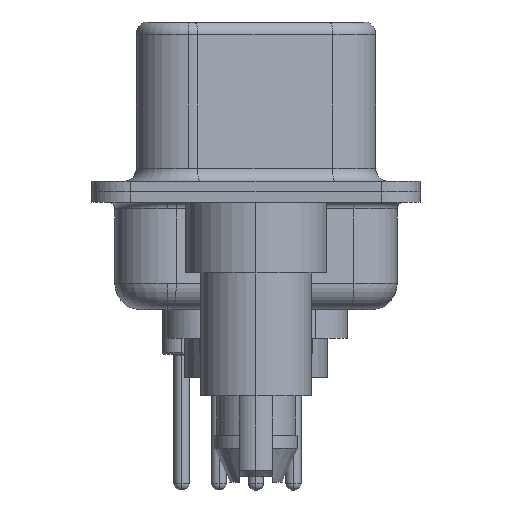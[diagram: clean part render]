
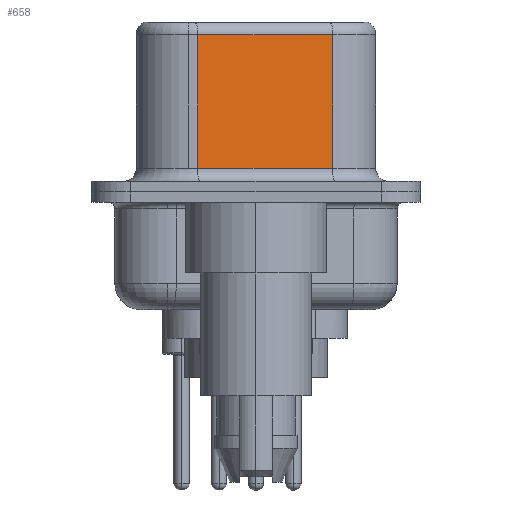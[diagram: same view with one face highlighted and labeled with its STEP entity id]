
A CAD part, left-side view. The second image highlights one B-rep face of the part: STEP entity #658.
In plain terms, the highlighted planar face has unit normal (-0.985, -0.174, 0).
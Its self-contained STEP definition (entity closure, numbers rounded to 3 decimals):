
#69 = VECTOR ( 'NONE', #6735, 1000. ) ;
#101 = DIRECTION ( 'NONE',  ( 0., 0., -1. ) ) ;
#658 = ADVANCED_FACE ( 'NONE', ( #16103 ), #24215, .F. ) ;
#712 = EDGE_CURVE ( 'NONE', #18961, #20043, #21652, .T. ) ;
#1178 = LINE ( 'NONE', #14080, #5476 ) ;
#2434 = EDGE_CURVE ( 'NONE', #5649, #19056, #1178, .T. ) ;
#4103 = ORIENTED_EDGE ( 'NONE', *, *, #13340, .T. ) ;
#4973 = DIRECTION ( 'NONE',  ( 0.985, 0.174, 0. ) ) ;
#5476 = VECTOR ( 'NONE', #24186, 1000. ) ;
#5649 = VERTEX_POINT ( 'NONE', #17119 ) ;
#6735 = DIRECTION ( 'NONE',  ( 0., 0., -1. ) ) ;
#8123 = ORIENTED_EDGE ( 'NONE', *, *, #2434, .T. ) ;
#8375 = CARTESIAN_POINT ( 'NONE',  ( 3.675, 2.233, 6.02 ) ) ;
#9322 = AXIS2_PLACEMENT_3D ( 'NONE', #12351, #4973, #10956 ) ;
#9620 = LINE ( 'NONE', #22506, #69 ) ;
#10956 = DIRECTION ( 'NONE',  ( -0.174, 0.985, 0. ) ) ;
#12351 = CARTESIAN_POINT ( 'NONE',  ( 4.585, -2.927, 6.52 ) ) ;
#13125 = EDGE_CURVE ( 'NONE', #5649, #20043, #9620, .T. ) ;
#13340 = EDGE_CURVE ( 'NONE', #19056, #18961, #17249, .T. ) ;
#14080 = CARTESIAN_POINT ( 'NONE',  ( 4.585, -2.927, 6.02 ) ) ;
#14487 = EDGE_LOOP ( 'NONE', ( #15422, #8123, #4103, #16860 ) ) ;
#15422 = ORIENTED_EDGE ( 'NONE', *, *, #13125, .F. ) ;
#15962 = CARTESIAN_POINT ( 'NONE',  ( 3.675, 2.233, 6.52 ) ) ;
#16103 = FACE_OUTER_BOUND ( 'NONE', #14487, .T. ) ;
#16288 = CARTESIAN_POINT ( 'NONE',  ( 4.585, -2.927, 0.9 ) ) ;
#16630 = CARTESIAN_POINT ( 'NONE',  ( 4.585, -2.927, 0.9 ) ) ;
#16860 = ORIENTED_EDGE ( 'NONE', *, *, #712, .T. ) ;
#17119 = CARTESIAN_POINT ( 'NONE',  ( 4.585, -2.927, 6.02 ) ) ;
#17249 = LINE ( 'NONE', #15962, #23709 ) ;
#18961 = VERTEX_POINT ( 'NONE', #20021 ) ;
#19056 = VERTEX_POINT ( 'NONE', #8375 ) ;
#20021 = CARTESIAN_POINT ( 'NONE',  ( 3.675, 2.233, 0.9 ) ) ;
#20043 = VERTEX_POINT ( 'NONE', #16288 ) ;
#21652 = LINE ( 'NONE', #16630, #24749 ) ;
#22506 = CARTESIAN_POINT ( 'NONE',  ( 4.585, -2.927, 6.52 ) ) ;
#22743 = DIRECTION ( 'NONE',  ( 0.174, -0.985, 0. ) ) ;
#23709 = VECTOR ( 'NONE', #101, 1000. ) ;
#24186 = DIRECTION ( 'NONE',  ( -0.174, 0.985, 0. ) ) ;
#24215 = PLANE ( 'NONE',  #9322 ) ;
#24749 = VECTOR ( 'NONE', #22743, 1000. ) ;
